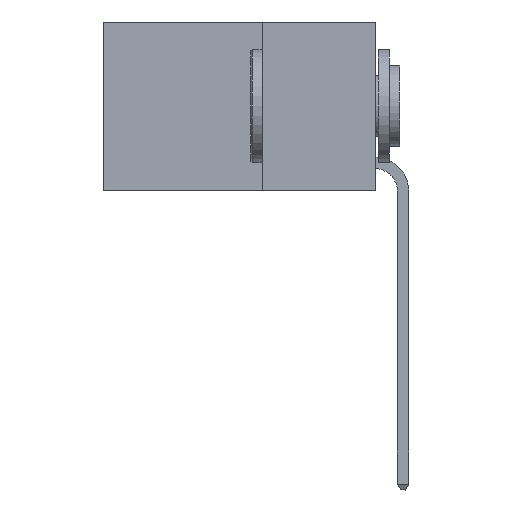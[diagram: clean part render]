
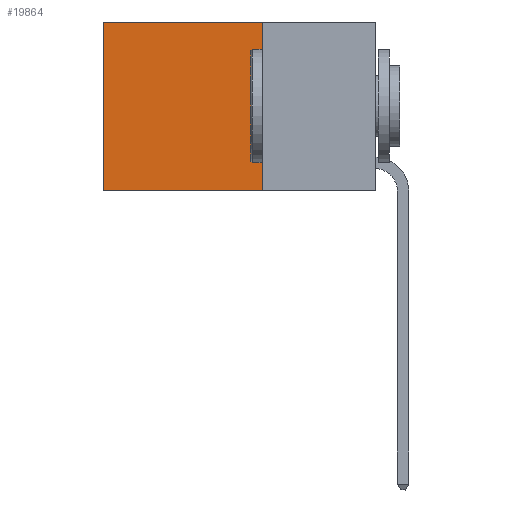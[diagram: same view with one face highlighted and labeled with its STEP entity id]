
A CAD part, left-side view. The second image highlights one B-rep face of the part: STEP entity #19864.
In plain terms, the highlighted planar face has unit normal (-1, 0, 0).
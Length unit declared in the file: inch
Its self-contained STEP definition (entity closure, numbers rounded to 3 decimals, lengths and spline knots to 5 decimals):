
#1276 = DIRECTION ( 'NONE',  ( 0., 0., -1. ) ) ;
#2074 = VERTEX_POINT ( 'NONE', #11424 ) ;
#2632 = EDGE_CURVE ( 'NONE', #12807, #20188, #12959, .T. ) ;
#3089 = EDGE_CURVE ( 'NONE', #12807, #2074, #5531, .T. ) ;
#4212 = VECTOR ( 'NONE', #18560, 39.37008 ) ;
#4717 = LINE ( 'NONE', #8404, #4212 ) ;
#5163 = VECTOR ( 'NONE', #8383, 39.37008 ) ;
#5531 = LINE ( 'NONE', #11380, #8434 ) ;
#6156 = ORIENTED_EDGE ( 'NONE', *, *, #3089, .F. ) ;
#6288 = PLANE ( 'NONE',  #12756 ) ;
#6696 = CARTESIAN_POINT ( 'NONE',  ( 0.2625, 0.25, -0.37 ) ) ;
#7971 = DIRECTION ( 'NONE',  ( 0., 0., -1. ) ) ;
#8199 = EDGE_CURVE ( 'NONE', #20188, #8788, #4717, .T. ) ;
#8233 = CARTESIAN_POINT ( 'NONE',  ( 0.2625, 0.6, -0.37 ) ) ;
#8383 = DIRECTION ( 'NONE',  ( 0., 1., 0. ) ) ;
#8404 = CARTESIAN_POINT ( 'NONE',  ( 0.2625, 0.6, 0. ) ) ;
#8434 = VECTOR ( 'NONE', #1276, 39.37008 ) ;
#8788 = VERTEX_POINT ( 'NONE', #8233 ) ;
#9201 = ORIENTED_EDGE ( 'NONE', *, *, #8199, .T. ) ;
#9678 = LINE ( 'NONE', #6696, #5163 ) ;
#9821 = CARTESIAN_POINT ( 'NONE',  ( 0.2625, 0.25, 0. ) ) ;
#9916 = EDGE_CURVE ( 'NONE', #2074, #8788, #9678, .T. ) ;
#10955 = EDGE_LOOP ( 'NONE', ( #9201, #18622, #6156, #17693 ) ) ;
#11380 = CARTESIAN_POINT ( 'NONE',  ( 0.2625, 0.25, 0. ) ) ;
#11424 = CARTESIAN_POINT ( 'NONE',  ( 0.2625, 0.25, -0.37 ) ) ;
#12756 = AXIS2_PLACEMENT_3D ( 'NONE', #19756, #18131, #7971 ) ;
#12807 = VERTEX_POINT ( 'NONE', #9821 ) ;
#12959 = LINE ( 'NONE', #19695, #16939 ) ;
#16939 = VECTOR ( 'NONE', #21067, 39.37008 ) ;
#17224 = CARTESIAN_POINT ( 'NONE',  ( 0.2625, 0.6, 0. ) ) ;
#17693 = ORIENTED_EDGE ( 'NONE', *, *, #2632, .T. ) ;
#18131 = DIRECTION ( 'NONE',  ( 1., 0., 0. ) ) ;
#18560 = DIRECTION ( 'NONE',  ( 0., 0., -1. ) ) ;
#18622 = ORIENTED_EDGE ( 'NONE', *, *, #9916, .F. ) ;
#19695 = CARTESIAN_POINT ( 'NONE',  ( 0.2625, 0.25, 0. ) ) ;
#19756 = CARTESIAN_POINT ( 'NONE',  ( 0.2625, 0.25, 0. ) ) ;
#19864 = ADVANCED_FACE ( 'NONE', ( #21579 ), #6288, .F. ) ;
#20188 = VERTEX_POINT ( 'NONE', #17224 ) ;
#21067 = DIRECTION ( 'NONE',  ( 0., 1., 0. ) ) ;
#21579 = FACE_OUTER_BOUND ( 'NONE', #10955, .T. ) ;
